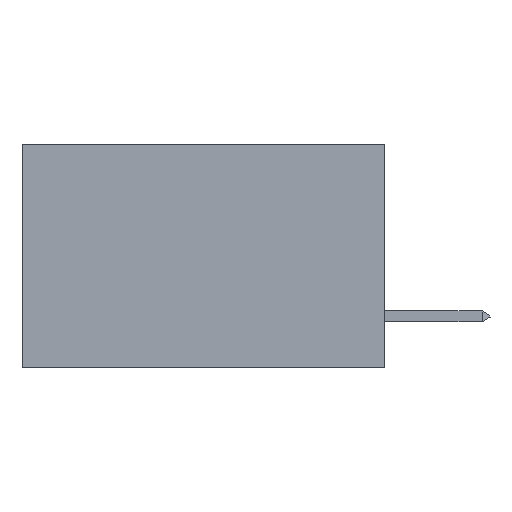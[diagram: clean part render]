
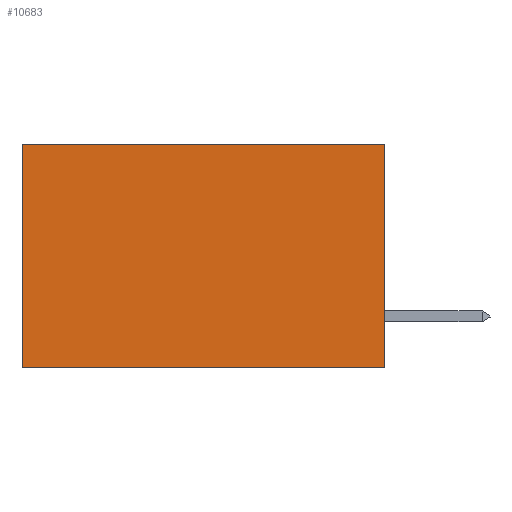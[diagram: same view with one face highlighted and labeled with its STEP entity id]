
A CAD part, left-side view. The second image highlights one B-rep face of the part: STEP entity #10683.
In plain terms, the highlighted planar face has unit normal (-1, 0, 0).
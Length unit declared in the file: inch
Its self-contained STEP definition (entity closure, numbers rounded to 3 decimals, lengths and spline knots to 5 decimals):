
#726 = EDGE_LOOP ( 'NONE', ( #10126, #22113, #12073, #1323 ) ) ;
#1122 = LINE ( 'NONE', #16253, #8144 ) ;
#1239 = CARTESIAN_POINT ( 'NONE',  ( 0.2875, 0., 0. ) ) ;
#1323 = ORIENTED_EDGE ( 'NONE', *, *, #6324, .T. ) ;
#1679 = VECTOR ( 'NONE', #13332, 39.37008 ) ;
#2652 = VERTEX_POINT ( 'NONE', #18756 ) ;
#2821 = DIRECTION ( 'NONE',  ( 0., 0., -1. ) ) ;
#5098 = DIRECTION ( 'NONE',  ( 0., 0., -1. ) ) ;
#5177 = AXIS2_PLACEMENT_3D ( 'NONE', #1239, #12977, #5098 ) ;
#5468 = EDGE_CURVE ( 'NONE', #2652, #5658, #1122, .T. ) ;
#5658 = VERTEX_POINT ( 'NONE', #20737 ) ;
#6324 = EDGE_CURVE ( 'NONE', #13787, #2652, #9942, .T. ) ;
#7640 = CARTESIAN_POINT ( 'NONE',  ( 0.2875, 0., -0.37 ) ) ;
#8109 = FACE_OUTER_BOUND ( 'NONE', #726, .T. ) ;
#8144 = VECTOR ( 'NONE', #2821, 39.37008 ) ;
#8917 = VERTEX_POINT ( 'NONE', #18183 ) ;
#9898 = LINE ( 'NONE', #13878, #19663 ) ;
#9942 = LINE ( 'NONE', #11028, #1679 ) ;
#10126 = ORIENTED_EDGE ( 'NONE', *, *, #5468, .T. ) ;
#10683 = ADVANCED_FACE ( 'NONE', ( #8109 ), #14936, .F. ) ;
#11028 = CARTESIAN_POINT ( 'NONE',  ( 0.2875, 0., 0. ) ) ;
#12073 = ORIENTED_EDGE ( 'NONE', *, *, #24542, .F. ) ;
#12977 = DIRECTION ( 'NONE',  ( 1., 0., 0. ) ) ;
#13332 = DIRECTION ( 'NONE',  ( 0., 1., 0. ) ) ;
#13787 = VERTEX_POINT ( 'NONE', #18580 ) ;
#13878 = CARTESIAN_POINT ( 'NONE',  ( 0.2875, 0., 0. ) ) ;
#14936 = PLANE ( 'NONE',  #5177 ) ;
#15515 = DIRECTION ( 'NONE',  ( 0., 1., 0. ) ) ;
#16253 = CARTESIAN_POINT ( 'NONE',  ( 0.2875, 0.6, 0. ) ) ;
#18183 = CARTESIAN_POINT ( 'NONE',  ( 0.2875, 0., -0.37 ) ) ;
#18315 = VECTOR ( 'NONE', #15515, 39.37008 ) ;
#18580 = CARTESIAN_POINT ( 'NONE',  ( 0.2875, 0., 0. ) ) ;
#18756 = CARTESIAN_POINT ( 'NONE',  ( 0.2875, 0.6, 0. ) ) ;
#19663 = VECTOR ( 'NONE', #21595, 39.37008 ) ;
#20737 = CARTESIAN_POINT ( 'NONE',  ( 0.2875, 0.6, -0.37 ) ) ;
#21252 = EDGE_CURVE ( 'NONE', #8917, #5658, #21305, .T. ) ;
#21305 = LINE ( 'NONE', #7640, #18315 ) ;
#21595 = DIRECTION ( 'NONE',  ( 0., 0., -1. ) ) ;
#22113 = ORIENTED_EDGE ( 'NONE', *, *, #21252, .F. ) ;
#24542 = EDGE_CURVE ( 'NONE', #13787, #8917, #9898, .T. ) ;
